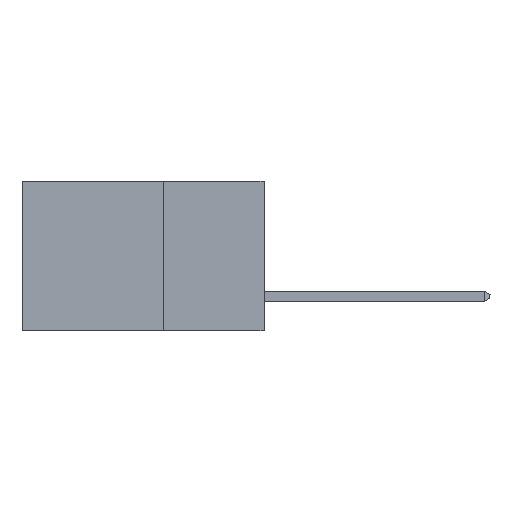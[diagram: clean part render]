
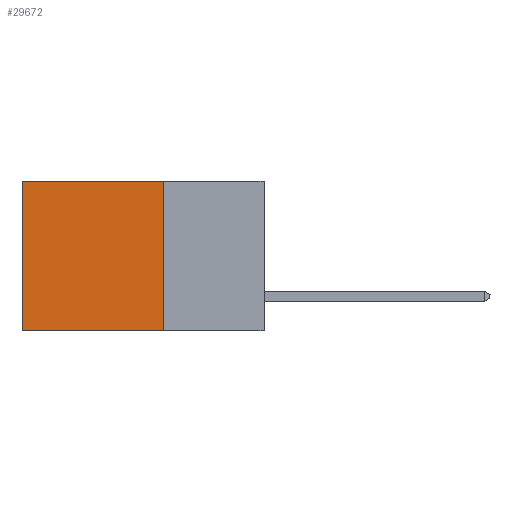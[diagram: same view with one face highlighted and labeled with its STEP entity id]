
A CAD part, left-side view. The second image highlights one B-rep face of the part: STEP entity #29672.
In plain terms, the highlighted planar face has unit normal (-1, 0, 0).
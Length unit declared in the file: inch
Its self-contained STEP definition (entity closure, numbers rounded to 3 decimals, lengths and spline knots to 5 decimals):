
#857 = LINE ( 'NONE', #14513, #6734 ) ;
#2117 = PLANE ( 'NONE',  #10466 ) ;
#2277 = VERTEX_POINT ( 'NONE', #28585 ) ;
#2284 = VECTOR ( 'NONE', #24981, 39.37008 ) ;
#3708 = ORIENTED_EDGE ( 'NONE', *, *, #12214, .F. ) ;
#4813 = VERTEX_POINT ( 'NONE', #14507 ) ;
#6153 = EDGE_CURVE ( 'NONE', #4813, #21943, #23730, .T. ) ;
#6212 = ORIENTED_EDGE ( 'NONE', *, *, #8797, .F. ) ;
#6734 = VECTOR ( 'NONE', #26390, 39.37008 ) ;
#7718 = CARTESIAN_POINT ( 'NONE',  ( 0.298, 0.25, 0. ) ) ;
#8797 = EDGE_CURVE ( 'NONE', #13588, #21943, #857, .T. ) ;
#10321 = CARTESIAN_POINT ( 'NONE',  ( 0.298, 0.25, 0. ) ) ;
#10466 = AXIS2_PLACEMENT_3D ( 'NONE', #18778, #11508, #13685 ) ;
#10848 = ORIENTED_EDGE ( 'NONE', *, *, #13184, .T. ) ;
#11508 = DIRECTION ( 'NONE',  ( 1., 0., 0. ) ) ;
#11574 = CARTESIAN_POINT ( 'NONE',  ( 0.298, 0.25, -0.37 ) ) ;
#12214 = EDGE_CURVE ( 'NONE', #2277, #13588, #28339, .T. ) ;
#13184 = EDGE_CURVE ( 'NONE', #2277, #4813, #20838, .T. ) ;
#13199 = DIRECTION ( 'NONE',  ( 0., 0., -1. ) ) ;
#13588 = VERTEX_POINT ( 'NONE', #11574 ) ;
#13685 = DIRECTION ( 'NONE',  ( 0., 0., -1. ) ) ;
#14507 = CARTESIAN_POINT ( 'NONE',  ( 0.298, 0.6, 0. ) ) ;
#14513 = CARTESIAN_POINT ( 'NONE',  ( 0.298, 0.25, -0.37 ) ) ;
#18778 = CARTESIAN_POINT ( 'NONE',  ( 0.298, 0.25, 0. ) ) ;
#20187 = EDGE_LOOP ( 'NONE', ( #30534, #6212, #3708, #10848 ) ) ;
#20676 = CARTESIAN_POINT ( 'NONE',  ( 0.298, 0.6, 0. ) ) ;
#20838 = LINE ( 'NONE', #7718, #24867 ) ;
#21320 = CARTESIAN_POINT ( 'NONE',  ( 0.298, 0.6, -0.37 ) ) ;
#21683 = DIRECTION ( 'NONE',  ( 0., 1., 0. ) ) ;
#21943 = VERTEX_POINT ( 'NONE', #21320 ) ;
#23730 = LINE ( 'NONE', #20676, #2284 ) ;
#24867 = VECTOR ( 'NONE', #21683, 39.37008 ) ;
#24981 = DIRECTION ( 'NONE',  ( 0., 0., -1. ) ) ;
#26390 = DIRECTION ( 'NONE',  ( 0., 1., 0. ) ) ;
#26518 = VECTOR ( 'NONE', #13199, 39.37008 ) ;
#28339 = LINE ( 'NONE', #10321, #26518 ) ;
#28585 = CARTESIAN_POINT ( 'NONE',  ( 0.298, 0.25, 0. ) ) ;
#29171 = FACE_OUTER_BOUND ( 'NONE', #20187, .T. ) ;
#29672 = ADVANCED_FACE ( 'NONE', ( #29171 ), #2117, .F. ) ;
#30534 = ORIENTED_EDGE ( 'NONE', *, *, #6153, .T. ) ;
